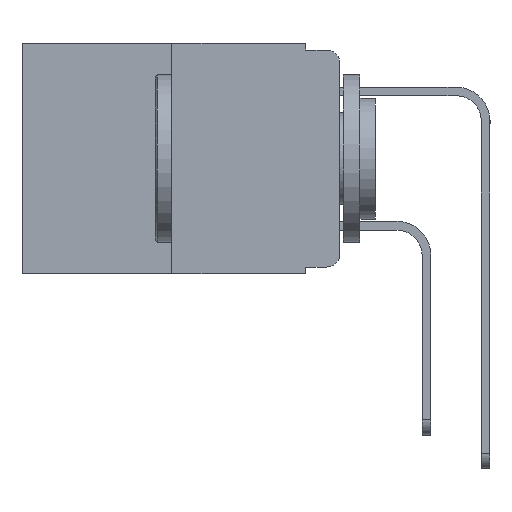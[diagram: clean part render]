
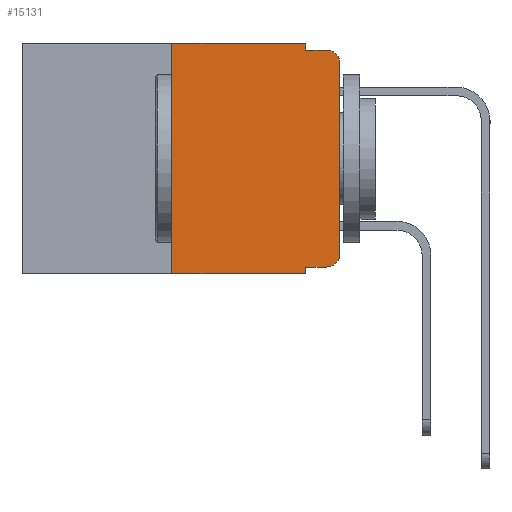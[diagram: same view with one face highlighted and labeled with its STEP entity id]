
A CAD part, left-side view. The second image highlights one B-rep face of the part: STEP entity #15131.
In plain terms, the highlighted planar face has unit normal (-1, 0, 0).
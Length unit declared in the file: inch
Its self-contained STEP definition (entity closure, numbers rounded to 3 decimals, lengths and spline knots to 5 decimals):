
#157 = AXIS2_PLACEMENT_3D ( 'NONE', #19305, #1902, #14199 ) ;
#166 = VERTEX_POINT ( 'NONE', #20867 ) ;
#1238 = EDGE_CURVE ( 'NONE', #6269, #15714, #20444, .T. ) ;
#1687 = VECTOR ( 'NONE', #7627, 39.37008 ) ;
#1693 = EDGE_CURVE ( 'NONE', #166, #6269, #7169, .T. ) ;
#1724 = VERTEX_POINT ( 'NONE', #9351 ) ;
#1902 = DIRECTION ( 'NONE',  ( 1., 0., 0. ) ) ;
#2179 = CARTESIAN_POINT ( 'NONE',  ( 0., 0.473, -0.343 ) ) ;
#2225 = DIRECTION ( 'NONE',  ( 0., -1., 0. ) ) ;
#2886 = VERTEX_POINT ( 'NONE', #12329 ) ;
#3322 = CARTESIAN_POINT ( 'NONE',  ( 0., 0.051, -0.01 ) ) ;
#4101 = EDGE_CURVE ( 'NONE', #18774, #166, #9488, .T. ) ;
#4672 = ORIENTED_EDGE ( 'NONE', *, *, #1693, .T. ) ;
#4871 = VECTOR ( 'NONE', #2225, 39.37008 ) ;
#5259 = ORIENTED_EDGE ( 'NONE', *, *, #21532, .T. ) ;
#5279 = EDGE_CURVE ( 'NONE', #18774, #1724, #14708, .T. ) ;
#5528 = AXIS2_PLACEMENT_3D ( 'NONE', #21457, #11126, #22473 ) ;
#5548 = CARTESIAN_POINT ( 'NONE',  ( 0., 0., -0.03 ) ) ;
#5870 = CARTESIAN_POINT ( 'NONE',  ( 0., 0.02, -0.03 ) ) ;
#5902 = DIRECTION ( 'NONE',  ( 0., -1., 0. ) ) ;
#5919 = CARTESIAN_POINT ( 'NONE',  ( 0., 0.25, 0. ) ) ;
#6269 = VERTEX_POINT ( 'NONE', #21847 ) ;
#6428 = LINE ( 'NONE', #5919, #1687 ) ;
#6609 = VECTOR ( 'NONE', #15621, 39.37008 ) ;
#6667 = LINE ( 'NONE', #17349, #15380 ) ;
#6844 = ORIENTED_EDGE ( 'NONE', *, *, #12168, .T. ) ;
#6849 = ORIENTED_EDGE ( 'NONE', *, *, #14663, .F. ) ;
#7169 = CIRCLE ( 'NONE', #5528, 0.02 ) ;
#7593 = DIRECTION ( 'NONE',  ( 0., 0., -1. ) ) ;
#7627 = DIRECTION ( 'NONE',  ( 0., 0., 1. ) ) ;
#7734 = CIRCLE ( 'NONE', #11802, 0.02 ) ;
#7833 = DIRECTION ( 'NONE',  ( 0., 0., -1. ) ) ;
#7968 = ORIENTED_EDGE ( 'NONE', *, *, #16931, .F. ) ;
#8648 = DIRECTION ( 'NONE',  ( 0., -1., 0. ) ) ;
#8770 = DIRECTION ( 'NONE',  ( 0., 0., -1. ) ) ;
#8772 = EDGE_CURVE ( 'NONE', #2886, #16025, #6667, .T. ) ;
#9289 = VECTOR ( 'NONE', #7833, 39.37008 ) ;
#9351 = CARTESIAN_POINT ( 'NONE',  ( 0., 0.051, -0.343 ) ) ;
#9488 = LINE ( 'NONE', #22221, #4871 ) ;
#9910 = FACE_OUTER_BOUND ( 'NONE', #18344, .T. ) ;
#10612 = LINE ( 'NONE', #2179, #20380 ) ;
#11126 = DIRECTION ( 'NONE',  ( -1., 0., 0. ) ) ;
#11802 = AXIS2_PLACEMENT_3D ( 'NONE', #5870, #17990, #7593 ) ;
#12168 = EDGE_CURVE ( 'NONE', #16480, #1724, #10612, .T. ) ;
#12329 = CARTESIAN_POINT ( 'NONE',  ( 0., 0.25, 0. ) ) ;
#12437 = PLANE ( 'NONE',  #157 ) ;
#12666 = ORIENTED_EDGE ( 'NONE', *, *, #8772, .F. ) ;
#13547 = CARTESIAN_POINT ( 'NONE',  ( 0., 0.25, -0.343 ) ) ;
#13739 = VERTEX_POINT ( 'NONE', #3322 ) ;
#13844 = CARTESIAN_POINT ( 'NONE',  ( 0., 0., 0. ) ) ;
#13983 = LINE ( 'NONE', #18242, #9289 ) ;
#14199 = DIRECTION ( 'NONE',  ( 0., 0., -1. ) ) ;
#14471 = DIRECTION ( 'NONE',  ( 0., -1., 0. ) ) ;
#14605 = CARTESIAN_POINT ( 'NONE',  ( 0., 0.051, -0.01 ) ) ;
#14663 = EDGE_CURVE ( 'NONE', #16480, #2886, #6428, .T. ) ;
#14708 = LINE ( 'NONE', #17467, #22191 ) ;
#15131 = ADVANCED_FACE ( 'NONE', ( #9910 ), #12437, .F. ) ;
#15380 = VECTOR ( 'NONE', #8648, 39.37008 ) ;
#15621 = DIRECTION ( 'NONE',  ( 0., 0., 1. ) ) ;
#15714 = VERTEX_POINT ( 'NONE', #5548 ) ;
#16025 = VERTEX_POINT ( 'NONE', #18591 ) ;
#16480 = VERTEX_POINT ( 'NONE', #13547 ) ;
#16931 = EDGE_CURVE ( 'NONE', #16025, #13739, #13983, .T. ) ;
#17088 = ORIENTED_EDGE ( 'NONE', *, *, #5279, .F. ) ;
#17349 = CARTESIAN_POINT ( 'NONE',  ( 0., 0.473, 0. ) ) ;
#17467 = CARTESIAN_POINT ( 'NONE',  ( 0., 0.051, 0. ) ) ;
#17760 = VERTEX_POINT ( 'NONE', #21493 ) ;
#17990 = DIRECTION ( 'NONE',  ( -1., 0., 0. ) ) ;
#18087 = LINE ( 'NONE', #14605, #21570 ) ;
#18242 = CARTESIAN_POINT ( 'NONE',  ( 0., 0.051, 0. ) ) ;
#18344 = EDGE_LOOP ( 'NONE', ( #22568, #5259, #20733, #7968, #12666, #6849, #6844, #17088, #20584, #4672 ) ) ;
#18591 = CARTESIAN_POINT ( 'NONE',  ( 0., 0.051, 0. ) ) ;
#18774 = VERTEX_POINT ( 'NONE', #20865 ) ;
#19305 = CARTESIAN_POINT ( 'NONE',  ( 0., 0.473, 0. ) ) ;
#20380 = VECTOR ( 'NONE', #14471, 39.37008 ) ;
#20406 = EDGE_CURVE ( 'NONE', #13739, #17760, #18087, .T. ) ;
#20444 = LINE ( 'NONE', #13844, #6609 ) ;
#20584 = ORIENTED_EDGE ( 'NONE', *, *, #4101, .T. ) ;
#20733 = ORIENTED_EDGE ( 'NONE', *, *, #20406, .F. ) ;
#20865 = CARTESIAN_POINT ( 'NONE',  ( 0., 0.051, -0.333 ) ) ;
#20867 = CARTESIAN_POINT ( 'NONE',  ( 0., 0.02, -0.333 ) ) ;
#21457 = CARTESIAN_POINT ( 'NONE',  ( 0., 0.02, -0.313 ) ) ;
#21493 = CARTESIAN_POINT ( 'NONE',  ( 0., 0.02, -0.01 ) ) ;
#21532 = EDGE_CURVE ( 'NONE', #15714, #17760, #7734, .T. ) ;
#21570 = VECTOR ( 'NONE', #5902, 39.37008 ) ;
#21847 = CARTESIAN_POINT ( 'NONE',  ( 0., 0., -0.313 ) ) ;
#22191 = VECTOR ( 'NONE', #8770, 39.37008 ) ;
#22221 = CARTESIAN_POINT ( 'NONE',  ( 0., 0.051, -0.333 ) ) ;
#22473 = DIRECTION ( 'NONE',  ( 0., 0., -1. ) ) ;
#22568 = ORIENTED_EDGE ( 'NONE', *, *, #1238, .T. ) ;
